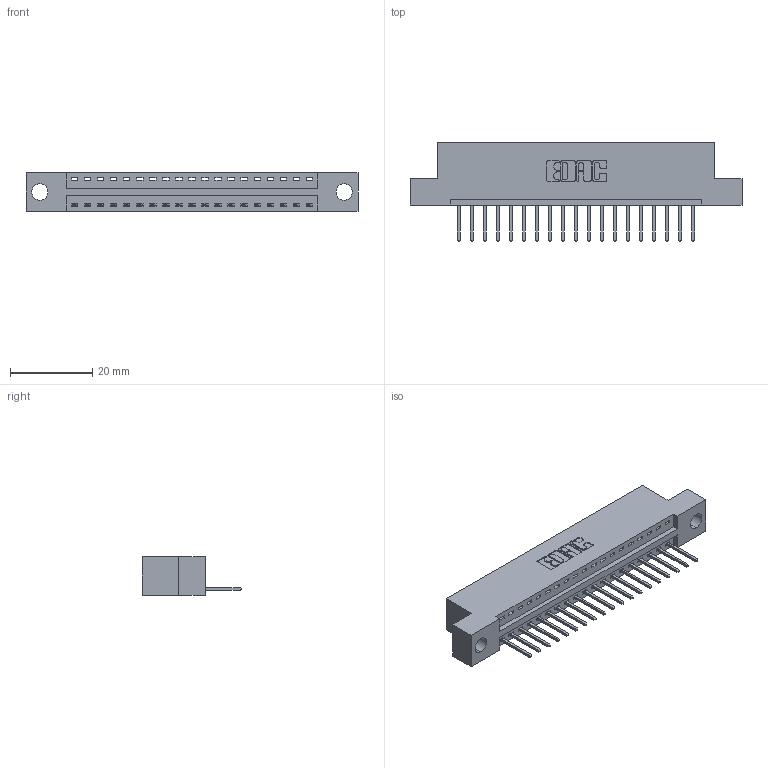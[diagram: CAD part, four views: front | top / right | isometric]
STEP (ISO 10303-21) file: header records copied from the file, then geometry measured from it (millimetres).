
FILE_DESCRIPTION (( 'STEP AP203' ), '1' );
FILE_NAME ('396-019-526-104.STEP', '2018-09-01T04:03:50', ( '' ), ( '' ), 'SwSTEP 2.0', 'SolidWorks 2016', '' );
FILE_SCHEMA (( 'CONFIG_CONTROL_DESIGN' ));
Length unit declared in the file: inch
Products named in the file (3): 346 Part_Flush Mounting Lugs - 0.156 Dia-TH; 345-292-001_345-293-126; 396-019-526-104
Assembly tree (20 placements, depth 2):
  396-019-526-104
    346 Part_Flush Mounting Lugs - 0.156 Dia-TH
    345-292-001_345-293-126  x19
Bounding box: 80.9 x 24.13 x 9.4 mm (x, y, z)
Volume: 7482.4 mm3; surface area: 8890.3 mm2
Topology: 20 solids, 20 shells, 1224 faces, 3673 edges, 2422 vertices
Faces by surface type: plane 836, cylinder 388
Entity records: 14909 total; most frequent: CARTESIAN_POINT 2569, ORIENTED_EDGE 2522, DIRECTION 2295, EDGE_CURVE 1261, LINE 1053, VECTOR 1053, VERTEX_POINT 838, AXIS2_PLACEMENT_3D 621
